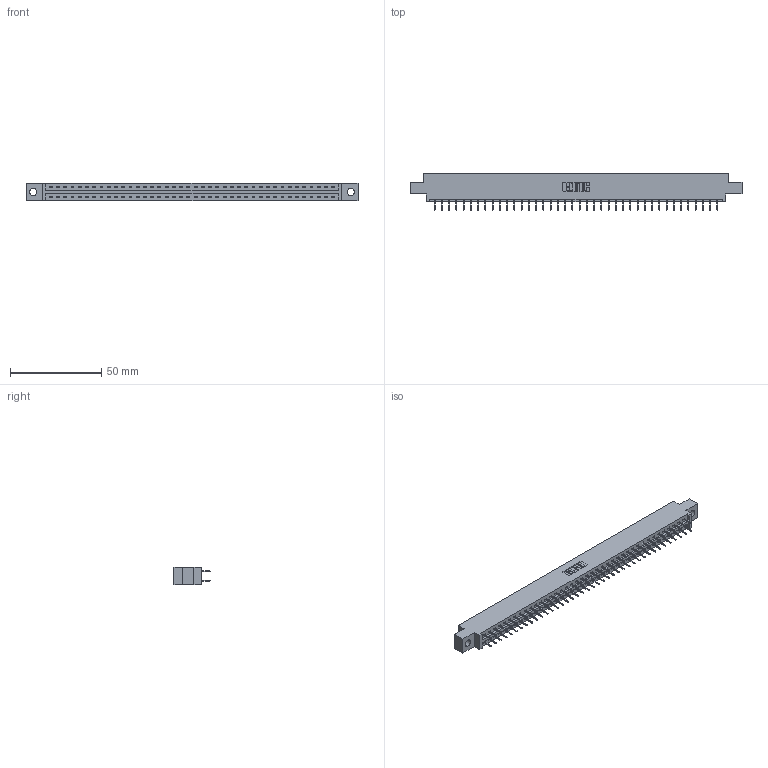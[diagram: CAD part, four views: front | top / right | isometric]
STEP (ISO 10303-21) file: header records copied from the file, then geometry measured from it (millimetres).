
FILE_DESCRIPTION (( 'STEP AP203' ), '1' );
FILE_NAME ('337-080-524-804.STEP', '2018-08-12T17:51:30', ( '' ), ( '' ), 'SwSTEP 2.0', 'SolidWorks 2016', '' );
FILE_SCHEMA (( 'CONFIG_CONTROL_DESIGN' ));
Length unit declared in the file: inch
Products named in the file (3): 337-080-524-804; 337 Part_0.170 Offset - 0.156 Dia-TH; 345-292-001_345-293-124
Assembly tree (81 placements, depth 2):
  337-080-524-804
    337 Part_0.170 Offset - 0.156 Dia-TH
    345-292-001_345-293-124  x80
Bounding box: 181.51 x 19.69 x 9.4 mm (x, y, z)
Volume: 18775.7 mm3; surface area: 20736.9 mm2
Topology: 81 solids, 81 shells, 4758 faces, 13523 edges, 8694 vertices
Faces by surface type: plane 3594, cylinder 1164
Entity records: 31481 total; most frequent: CARTESIAN_POINT 5306, ORIENTED_EDGE 5242, DIRECTION 4517, EDGE_CURVE 2621, LINE 2497, VECTOR 2497, VERTEX_POINT 1742, AXIS2_PLACEMENT_3D 1010
